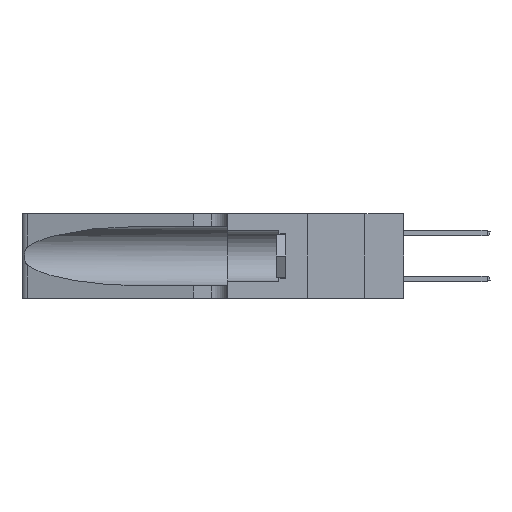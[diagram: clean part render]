
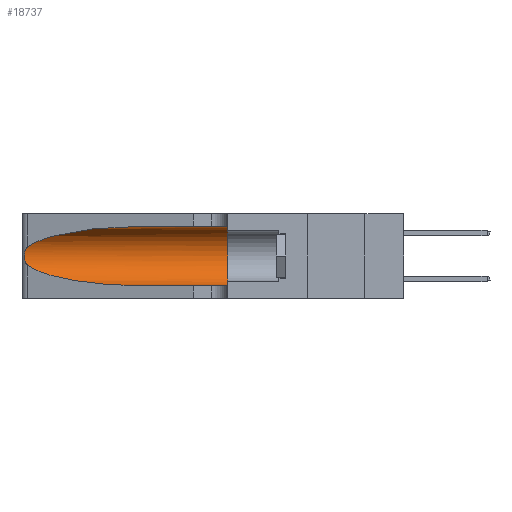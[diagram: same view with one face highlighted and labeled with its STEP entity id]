
A CAD part, left-side view. The second image highlights one B-rep face of the part: STEP entity #18737.
In plain terms, the highlighted cylindrical face has radius 3.308 mm (diameter 6.617 mm), a partial arc.
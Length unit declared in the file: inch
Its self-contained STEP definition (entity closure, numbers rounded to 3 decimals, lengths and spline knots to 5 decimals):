
#127 = CARTESIAN_POINT ( 'NONE',  ( 0.18966, 0.96281, 0.05475 ) ) ;
#515 = CARTESIAN_POINT ( 'NONE',  ( 0.1305, 1.61858, 0.05475 ) ) ;
#2334 = CARTESIAN_POINT ( 'NONE',  ( 0.25856, 1.23593, 0.16098 ) ) ;
#2665 = CARTESIAN_POINT ( 'NONE',  ( 0.1305, 0.72297, 0.05475 ) ) ;
#4756 = CARTESIAN_POINT ( 'NONE',  ( 0.25787, 1.23484, 0.2124 ) ) ;
#5090 =( BOUNDED_CURVE ( )  B_SPLINE_CURVE ( 3, ( #5318, #14972, #127, #2665 ),
 .UNSPECIFIED., .F., .F. ) 
 B_SPLINE_CURVE_WITH_KNOTS ( ( 4, 4 ),
 ( 3.44316, 4.71239 ),
 .UNSPECIFIED. ) 
 CURVE ( )  GEOMETRIC_REPRESENTATION_ITEM ( )  RATIONAL_B_SPLINE_CURVE ( ( 1., 0.87, 0.87, 1. ) ) 
 REPRESENTATION_ITEM ( '' )  );
#5131 = EDGE_CURVE ( 'NONE', #7318, #7330, #5090, .T. ) ;
#5305 = VERTEX_POINT ( 'NONE', #13619 ) ;
#5318 = CARTESIAN_POINT ( 'NONE',  ( 0.25487, 1.22718, 0.14631 ) ) ;
#7318 = VERTEX_POINT ( 'NONE', #23210 ) ;
#7330 = VERTEX_POINT ( 'NONE', #21983 ) ;
#7409 = DIRECTION ( 'NONE',  ( 0., -1., 0. ) ) ;
#7411 = CARTESIAN_POINT ( 'NONE',  ( 0.25487, 1.22718, 0.22369 ) ) ;
#7628 = CARTESIAN_POINT ( 'NONE',  ( 0.1305, 1.61858, 0.185 ) ) ;
#7629 = CARTESIAN_POINT ( 'NONE',  ( 0.25555, 1.22993, 0.14849 ) ) ;
#8811 = LINE ( 'NONE', #17168, #16255 ) ;
#9106 = EDGE_CURVE ( 'NONE', #31980, #20587, #8811, .T. ) ;
#9434 = EDGE_CURVE ( 'NONE', #31980, #5305, #16368, .T. ) ;
#10067 = CARTESIAN_POINT ( 'NONE',  ( 0.1305, 0.35, 0.05475 ) ) ;
#10211 = ORIENTED_EDGE ( 'NONE', *, *, #12869, .F. ) ;
#11353 = FACE_OUTER_BOUND ( 'NONE', #27140, .T. ) ;
#11909 = ORIENTED_EDGE ( 'NONE', *, *, #26933, .T. ) ;
#12558 = CARTESIAN_POINT ( 'NONE',  ( 0.26075, 1.23896, 0.19203 ) ) ;
#12703 = DIRECTION ( 'NONE',  ( 0., 0., 1. ) ) ;
#12869 = EDGE_CURVE ( 'NONE', #20587, #21845, #28688, .T. ) ;
#12942 = CARTESIAN_POINT ( 'NONE',  ( 0.25487, 1.22718, 0.22369 ) ) ;
#13619 = CARTESIAN_POINT ( 'NONE',  ( 0.25487, 1.22718, 0.22369 ) ) ;
#14870 = CARTESIAN_POINT ( 'NONE',  ( 0.26018, 1.23835, 0.19895 ) ) ;
#14971 = CARTESIAN_POINT ( 'NONE',  ( 0.25854, 1.2359, 0.20912 ) ) ;
#14972 = CARTESIAN_POINT ( 'NONE',  ( 0.2373, 1.15595, 0.08982 ) ) ;
#15088 = CARTESIAN_POINT ( 'NONE',  ( 0.25789, 1.23486, 0.15765 ) ) ;
#15661 = AXIS2_PLACEMENT_3D ( 'NONE', #22778, #27647, #12703 ) ;
#16255 = VECTOR ( 'NONE', #30633, 39.37008 ) ;
#16368 =( BOUNDED_CURVE ( )  B_SPLINE_CURVE ( 3, ( #23538, #18444, #20684, #12942 ),
 .UNSPECIFIED., .F., .F. ) 
 B_SPLINE_CURVE_WITH_KNOTS ( ( 4, 4 ),
 ( 1.5708, 2.84003 ),
 .UNSPECIFIED. ) 
 CURVE ( )  GEOMETRIC_REPRESENTATION_ITEM ( )  RATIONAL_B_SPLINE_CURVE ( ( 1., 0.87, 0.87, 1. ) ) 
 REPRESENTATION_ITEM ( '' )  );
#17168 = CARTESIAN_POINT ( 'NONE',  ( 0.1305, 1.61858, 0.31525 ) ) ;
#17249 = ORIENTED_EDGE ( 'NONE', *, *, #27750, .T. ) ;
#17289 = LINE ( 'NONE', #515, #22420 ) ;
#17300 = CARTESIAN_POINT ( 'NONE',  ( 0.25555, 1.22994, 0.2215 ) ) ;
#17524 = CARTESIAN_POINT ( 'NONE',  ( 0.25639, 1.23184, 0.21858 ) ) ;
#18444 = CARTESIAN_POINT ( 'NONE',  ( 0.18966, 0.96281, 0.31525 ) ) ;
#18737 = ADVANCED_FACE ( 'NONE', ( #11353 ), #25151, .F. ) ;
#19567 = AXIS2_PLACEMENT_3D ( 'NONE', #7628, #7409, #27607 ) ;
#20231 = CARTESIAN_POINT ( 'NONE',  ( 0.1305, 0.35, 0.31525 ) ) ;
#20587 = VERTEX_POINT ( 'NONE', #20231 ) ;
#20684 = CARTESIAN_POINT ( 'NONE',  ( 0.2373, 1.15595, 0.28018 ) ) ;
#21302 = ORIENTED_EDGE ( 'NONE', *, *, #9434, .T. ) ;
#21374 = ORIENTED_EDGE ( 'NONE', *, *, #9106, .F. ) ;
#21845 = VERTEX_POINT ( 'NONE', #10067 ) ;
#21983 = CARTESIAN_POINT ( 'NONE',  ( 0.1305, 0.72297, 0.05475 ) ) ;
#22420 = VECTOR ( 'NONE', #28234, 39.37008 ) ;
#22521 = CARTESIAN_POINT ( 'NONE',  ( 0.25639, 1.23186, 0.15144 ) ) ;
#22736 = CARTESIAN_POINT ( 'NONE',  ( 0.26017, 1.23833, 0.17102 ) ) ;
#22778 = CARTESIAN_POINT ( 'NONE',  ( 0.1305, 0.35, 0.185 ) ) ;
#23210 = CARTESIAN_POINT ( 'NONE',  ( 0.25487, 1.22718, 0.14631 ) ) ;
#23538 = CARTESIAN_POINT ( 'NONE',  ( 0.1305, 0.72297, 0.31525 ) ) ;
#24439 = CARTESIAN_POINT ( 'NONE',  ( 0.1305, 0.72297, 0.31525 ) ) ;
#24797 = ORIENTED_EDGE ( 'NONE', *, *, #5131, .T. ) ;
#25047 = CARTESIAN_POINT ( 'NONE',  ( 0.25487, 1.22718, 0.14631 ) ) ;
#25151 = CYLINDRICAL_SURFACE ( 'NONE', #19567, 0.13025 ) ;
#26933 = EDGE_CURVE ( 'NONE', #5305, #7318, #27549, .T. ) ;
#27140 = EDGE_LOOP ( 'NONE', ( #21302, #11909, #24797, #17249, #10211, #21374 ) ) ;
#27549 = B_SPLINE_CURVE_WITH_KNOTS ( 'NONE', 3,
 ( #7411, #17300, #17524, #4756, #14971, #14870, #12558, #32556, #22736, #2334, #15088, #22521, #7629, #25047 ),
 .UNSPECIFIED., .F., .F.,
 ( 4, 2, 2, 2, 2, 2, 4 ),
 ( 0., 0.00027, 0.00053, 0.00107, 0.0016, 0.00187, 0.00214 ),
 .UNSPECIFIED. ) ;
#27607 = DIRECTION ( 'NONE',  ( 0., 0., -1. ) ) ;
#27647 = DIRECTION ( 'NONE',  ( 0., 1., 0. ) ) ;
#27750 = EDGE_CURVE ( 'NONE', #7330, #21845, #17289, .T. ) ;
#28234 = DIRECTION ( 'NONE',  ( 0., -1., 0. ) ) ;
#28688 = CIRCLE ( 'NONE', #15661, 0.13025 ) ;
#30633 = DIRECTION ( 'NONE',  ( 0., -1., 0. ) ) ;
#31980 = VERTEX_POINT ( 'NONE', #24439 ) ;
#32556 = CARTESIAN_POINT ( 'NONE',  ( 0.26075, 1.23896, 0.178 ) ) ;
